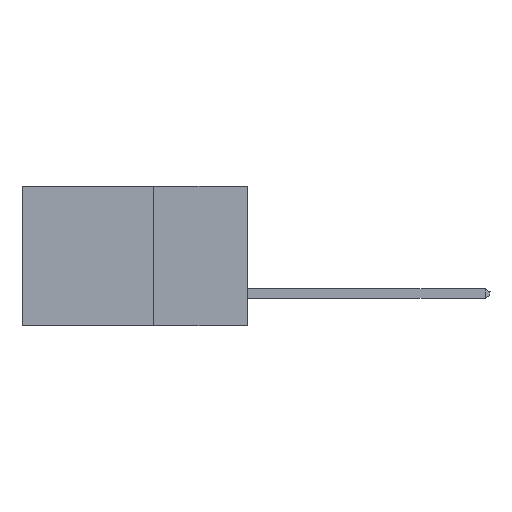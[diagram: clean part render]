
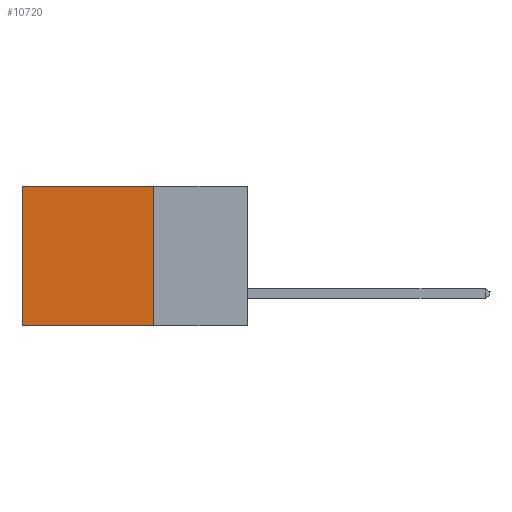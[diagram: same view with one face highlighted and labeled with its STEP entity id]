
A CAD part, left-side view. The second image highlights one B-rep face of the part: STEP entity #10720.
In plain terms, the highlighted planar face has unit normal (-1, 0, 0).
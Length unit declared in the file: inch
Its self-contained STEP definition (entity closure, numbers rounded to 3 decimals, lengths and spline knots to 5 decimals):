
#1998 = DIRECTION ( 'NONE',  ( 0., 0., -1. ) ) ;
#2104 = DIRECTION ( 'NONE',  ( 0., 1., 0. ) ) ;
#2255 = LINE ( 'NONE', #21785, #7301 ) ;
#2257 = EDGE_LOOP ( 'NONE', ( #8175, #20411, #25564, #5323 ) ) ;
#2782 = DIRECTION ( 'NONE',  ( 0., 1., 0. ) ) ;
#3856 = VERTEX_POINT ( 'NONE', #24337 ) ;
#4843 = CARTESIAN_POINT ( 'NONE',  ( 0.2615, 0.25, -0.37 ) ) ;
#4867 = LINE ( 'NONE', #16846, #8953 ) ;
#5092 = FACE_OUTER_BOUND ( 'NONE', #2257, .T. ) ;
#5323 = ORIENTED_EDGE ( 'NONE', *, *, #6667, .T. ) ;
#6667 = EDGE_CURVE ( 'NONE', #17006, #3856, #10445, .T. ) ;
#6782 = CARTESIAN_POINT ( 'NONE',  ( 0.2615, 0.25, -0.37 ) ) ;
#7301 = VECTOR ( 'NONE', #1998, 39.37008 ) ;
#8175 = ORIENTED_EDGE ( 'NONE', *, *, #22142, .T. ) ;
#8953 = VECTOR ( 'NONE', #24649, 39.37008 ) ;
#9005 = DIRECTION ( 'NONE',  ( 1., 0., 0. ) ) ;
#10445 = LINE ( 'NONE', #10841, #22626 ) ;
#10720 = ADVANCED_FACE ( 'NONE', ( #5092 ), #13173, .F. ) ;
#10841 = CARTESIAN_POINT ( 'NONE',  ( 0.2615, 0.25, 0. ) ) ;
#11923 = AXIS2_PLACEMENT_3D ( 'NONE', #4843, #9005, #16704 ) ;
#12237 = VERTEX_POINT ( 'NONE', #20068 ) ;
#13173 = PLANE ( 'NONE',  #11923 ) ;
#16704 = DIRECTION ( 'NONE',  ( 0., 0., -1. ) ) ;
#16730 = VERTEX_POINT ( 'NONE', #6782 ) ;
#16846 = CARTESIAN_POINT ( 'NONE',  ( 0.2615, 0.6, -0.37 ) ) ;
#17006 = VERTEX_POINT ( 'NONE', #17697 ) ;
#17697 = CARTESIAN_POINT ( 'NONE',  ( 0.2615, 0.25, 0. ) ) ;
#17868 = CARTESIAN_POINT ( 'NONE',  ( 0.2615, 0.25, -0.37 ) ) ;
#20068 = CARTESIAN_POINT ( 'NONE',  ( 0.2615, 0.6, -0.37 ) ) ;
#20208 = LINE ( 'NONE', #17868, #20965 ) ;
#20411 = ORIENTED_EDGE ( 'NONE', *, *, #21107, .F. ) ;
#20965 = VECTOR ( 'NONE', #2104, 39.37008 ) ;
#21107 = EDGE_CURVE ( 'NONE', #16730, #12237, #20208, .T. ) ;
#21785 = CARTESIAN_POINT ( 'NONE',  ( 0.2615, 0.25, -0.37 ) ) ;
#22142 = EDGE_CURVE ( 'NONE', #3856, #12237, #4867, .T. ) ;
#22626 = VECTOR ( 'NONE', #2782, 39.37008 ) ;
#24294 = EDGE_CURVE ( 'NONE', #17006, #16730, #2255, .T. ) ;
#24337 = CARTESIAN_POINT ( 'NONE',  ( 0.2615, 0.6, 0. ) ) ;
#24649 = DIRECTION ( 'NONE',  ( 0., 0., -1. ) ) ;
#25564 = ORIENTED_EDGE ( 'NONE', *, *, #24294, .F. ) ;
